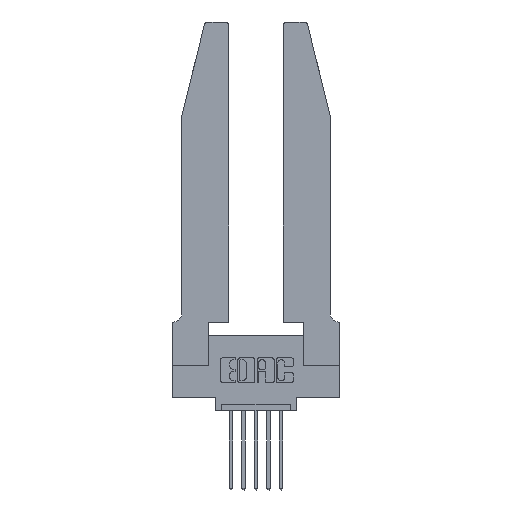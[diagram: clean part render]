
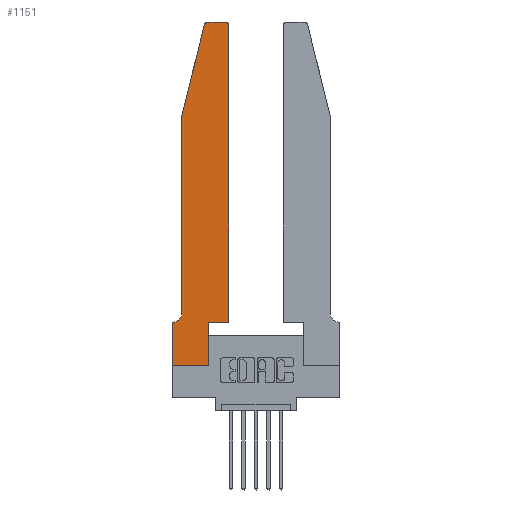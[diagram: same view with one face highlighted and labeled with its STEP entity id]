
A CAD part, top view. The second image highlights one B-rep face of the part: STEP entity #1151.
In plain terms, the highlighted planar face has unit normal (0, 0, 1).
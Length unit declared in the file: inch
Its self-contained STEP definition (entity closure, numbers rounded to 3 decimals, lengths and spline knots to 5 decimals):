
#177 = EDGE_CURVE ( 'NONE', #4136, #11993, #3671, .T. ) ;
#234 = DIRECTION ( 'NONE',  ( 0., -1., 0. ) ) ;
#373 = DIRECTION ( 'NONE',  ( -1., 0., 0. ) ) ;
#794 = CARTESIAN_POINT ( 'NONE',  ( 0.2865, 0., 0.37 ) ) ;
#994 = ORIENTED_EDGE ( 'NONE', *, *, #177, .T. ) ;
#1151 = ADVANCED_FACE ( 'NONE', ( #2000 ), #3308, .T. ) ;
#1167 = ORIENTED_EDGE ( 'NONE', *, *, #3946, .T. ) ;
#1638 = DIRECTION ( 'NONE',  ( -1., 0., 0. ) ) ;
#1746 = DIRECTION ( 'NONE',  ( 1., 0., 0. ) ) ;
#1855 = VECTOR ( 'NONE', #234, 39.37008 ) ;
#2000 = FACE_OUTER_BOUND ( 'NONE', #8129, .T. ) ;
#2138 = VECTOR ( 'NONE', #7145, 39.37008 ) ;
#2608 = CARTESIAN_POINT ( 'NONE',  ( 0.284, 2.72, 0.37 ) ) ;
#2638 = CARTESIAN_POINT ( 'NONE',  ( 0.0755, 2., 0.37 ) ) ;
#2796 = VECTOR ( 'NONE', #4266, 39.37008 ) ;
#3174 = EDGE_CURVE ( 'NONE', #3297, #4732, #5863, .T. ) ;
#3292 = ORIENTED_EDGE ( 'NONE', *, *, #10924, .T. ) ;
#3297 = VERTEX_POINT ( 'NONE', #11912 ) ;
#3308 = PLANE ( 'NONE',  #7820 ) ;
#3459 = VERTEX_POINT ( 'NONE', #10977 ) ;
#3528 = ORIENTED_EDGE ( 'NONE', *, *, #8869, .T. ) ;
#3563 = AXIS2_PLACEMENT_3D ( 'NONE', #2608, #6756, #12046 ) ;
#3671 = LINE ( 'NONE', #3792, #11635 ) ;
#3792 = CARTESIAN_POINT ( 'NONE',  ( 0., 0., 0.37 ) ) ;
#3946 = EDGE_CURVE ( 'NONE', #3459, #10819, #10806, .T. ) ;
#4136 = VERTEX_POINT ( 'NONE', #8554 ) ;
#4266 = DIRECTION ( 'NONE',  ( 0., 1., 0. ) ) ;
#4281 = CIRCLE ( 'NONE', #11032, 0.03 ) ;
#4580 = CARTESIAN_POINT ( 'NONE',  ( 0.4505, 0.35, 0.37 ) ) ;
#4597 = ORIENTED_EDGE ( 'NONE', *, *, #3174, .T. ) ;
#4599 = VECTOR ( 'NONE', #1638, 39.37008 ) ;
#4661 = ORIENTED_EDGE ( 'NONE', *, *, #12497, .T. ) ;
#4732 = VERTEX_POINT ( 'NONE', #2638 ) ;
#4739 = LINE ( 'NONE', #10587, #2796 ) ;
#5197 = VERTEX_POINT ( 'NONE', #5598 ) ;
#5433 = LINE ( 'NONE', #12344, #2138 ) ;
#5598 = CARTESIAN_POINT ( 'NONE',  ( 0.4205, 2.75, 0.37 ) ) ;
#5665 = DIRECTION ( 'NONE',  ( 0., 0., -1. ) ) ;
#5764 = CARTESIAN_POINT ( 'NONE',  ( 0.4505, 2.72, 0.37 ) ) ;
#5863 = LINE ( 'NONE', #6777, #8040 ) ;
#5874 = CARTESIAN_POINT ( 'NONE',  ( 0.0055, 0.35, 0.37 ) ) ;
#6094 = EDGE_CURVE ( 'NONE', #8137, #4136, #11774, .T. ) ;
#6227 = ORIENTED_EDGE ( 'NONE', *, *, #6896, .T. ) ;
#6437 = VECTOR ( 'NONE', #6470, 39.37008 ) ;
#6439 = ORIENTED_EDGE ( 'NONE', *, *, #6094, .T. ) ;
#6470 = DIRECTION ( 'NONE',  ( 0., 1., 0. ) ) ;
#6756 = DIRECTION ( 'NONE',  ( 0., 0., 1. ) ) ;
#6777 = CARTESIAN_POINT ( 'NONE',  ( 0.0755, 2., 0.37 ) ) ;
#6838 = CARTESIAN_POINT ( 'NONE',  ( 0.4505, 0.35, 0.37 ) ) ;
#6896 = EDGE_CURVE ( 'NONE', #10819, #8137, #7433, .T. ) ;
#7145 = DIRECTION ( 'NONE',  ( 0., -1., 0. ) ) ;
#7216 = DIRECTION ( 'NONE',  ( 1., 0., 0. ) ) ;
#7433 = LINE ( 'NONE', #10887, #4599 ) ;
#7508 = CARTESIAN_POINT ( 'NONE',  ( 0.2605, 2.75, 0.37 ) ) ;
#7556 = DIRECTION ( 'NONE',  ( -1., 0., 0. ) ) ;
#7620 = EDGE_CURVE ( 'NONE', #9902, #5197, #4281, .T. ) ;
#7811 = DIRECTION ( 'NONE',  ( 1., 0., 0. ) ) ;
#7820 = AXIS2_PLACEMENT_3D ( 'NONE', #10639, #8561, #10504 ) ;
#8040 = VECTOR ( 'NONE', #10869, 39.37008 ) ;
#8129 = EDGE_LOOP ( 'NONE', ( #3528, #4661, #4597, #10345, #1167, #6227, #6439, #994, #9295, #3292, #12842, #10891 ) ) ;
#8137 = VERTEX_POINT ( 'NONE', #10686 ) ;
#8554 = CARTESIAN_POINT ( 'NONE',  ( 0., 0., 0.37 ) ) ;
#8561 = DIRECTION ( 'NONE',  ( 0., 0., 1. ) ) ;
#8597 = CARTESIAN_POINT ( 'NONE',  ( 0., 0., 0.37 ) ) ;
#8869 = EDGE_CURVE ( 'NONE', #5197, #12770, #9338, .T. ) ;
#9295 = ORIENTED_EDGE ( 'NONE', *, *, #12413, .T. ) ;
#9338 = LINE ( 'NONE', #7508, #10801 ) ;
#9620 = VECTOR ( 'NONE', #7811, 39.37008 ) ;
#9902 = VERTEX_POINT ( 'NONE', #5764 ) ;
#10219 = CARTESIAN_POINT ( 'NONE',  ( 0.2865, 0.35, 0.37 ) ) ;
#10340 = DIRECTION ( 'NONE',  ( 0., 0., 1. ) ) ;
#10345 = ORIENTED_EDGE ( 'NONE', *, *, #11705, .T. ) ;
#10504 = DIRECTION ( 'NONE',  ( 1., 0., 0. ) ) ;
#10587 = CARTESIAN_POINT ( 'NONE',  ( 0.2865, 0.35, 0.37 ) ) ;
#10639 = CARTESIAN_POINT ( 'NONE',  ( 0., 0.35, 0.37 ) ) ;
#10650 = CARTESIAN_POINT ( 'NONE',  ( 0.4505, 0.35, 0.37 ) ) ;
#10686 = CARTESIAN_POINT ( 'NONE',  ( 0., 0.35, 0.37 ) ) ;
#10801 = VECTOR ( 'NONE', #7556, 39.37008 ) ;
#10806 = CIRCLE ( 'NONE', #12785, 0.07 ) ;
#10819 = VERTEX_POINT ( 'NONE', #5874 ) ;
#10869 = DIRECTION ( 'NONE',  ( -0.239, -0.971, 0. ) ) ;
#10887 = CARTESIAN_POINT ( 'NONE',  ( 0.0755, 0.35, 0.37 ) ) ;
#10891 = ORIENTED_EDGE ( 'NONE', *, *, #7620, .T. ) ;
#10924 = EDGE_CURVE ( 'NONE', #11685, #11978, #12924, .T. ) ;
#10956 = CARTESIAN_POINT ( 'NONE',  ( 0.0055, 0.42, 0.37 ) ) ;
#10977 = CARTESIAN_POINT ( 'NONE',  ( 0.0755, 0.42, 0.37 ) ) ;
#11032 = AXIS2_PLACEMENT_3D ( 'NONE', #13572, #10340, #7216 ) ;
#11414 = LINE ( 'NONE', #10650, #6437 ) ;
#11611 = CARTESIAN_POINT ( 'NONE',  ( 0.284, 2.75, 0.37 ) ) ;
#11635 = VECTOR ( 'NONE', #1746, 39.37008 ) ;
#11685 = VERTEX_POINT ( 'NONE', #10219 ) ;
#11705 = EDGE_CURVE ( 'NONE', #4732, #3459, #5433, .T. ) ;
#11774 = LINE ( 'NONE', #8597, #1855 ) ;
#11912 = CARTESIAN_POINT ( 'NONE',  ( 0.25487, 2.72718, 0.37 ) ) ;
#11978 = VERTEX_POINT ( 'NONE', #6838 ) ;
#11993 = VERTEX_POINT ( 'NONE', #794 ) ;
#12046 = DIRECTION ( 'NONE',  ( 1., 0., 0. ) ) ;
#12208 = EDGE_CURVE ( 'NONE', #11978, #9902, #11414, .T. ) ;
#12344 = CARTESIAN_POINT ( 'NONE',  ( 0.0755, 2., 0.37 ) ) ;
#12413 = EDGE_CURVE ( 'NONE', #11993, #11685, #4739, .T. ) ;
#12497 = EDGE_CURVE ( 'NONE', #12770, #3297, #13040, .T. ) ;
#12770 = VERTEX_POINT ( 'NONE', #11611 ) ;
#12785 = AXIS2_PLACEMENT_3D ( 'NONE', #10956, #5665, #373 ) ;
#12842 = ORIENTED_EDGE ( 'NONE', *, *, #12208, .T. ) ;
#12924 = LINE ( 'NONE', #4580, #9620 ) ;
#13040 = CIRCLE ( 'NONE', #3563, 0.03 ) ;
#13572 = CARTESIAN_POINT ( 'NONE',  ( 0.4205, 2.72, 0.37 ) ) ;
